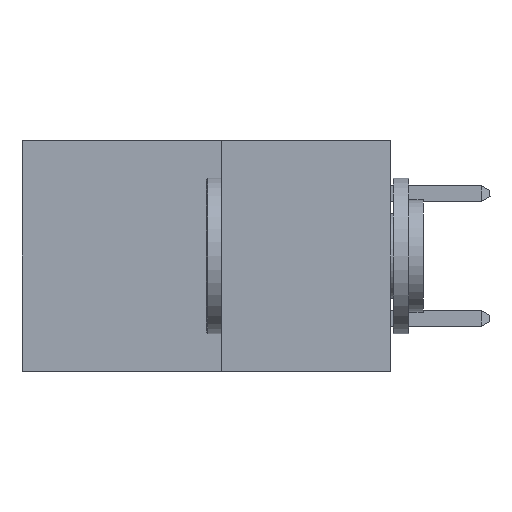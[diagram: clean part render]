
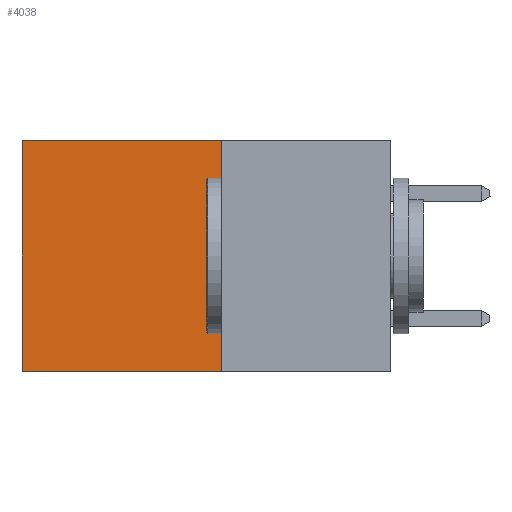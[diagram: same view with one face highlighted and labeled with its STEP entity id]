
A CAD part, left-side view. The second image highlights one B-rep face of the part: STEP entity #4038.
In plain terms, the highlighted planar face has unit normal (-1, 0, 0).
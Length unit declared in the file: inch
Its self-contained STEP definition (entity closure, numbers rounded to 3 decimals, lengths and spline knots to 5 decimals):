
#106 = CARTESIAN_POINT ( 'NONE',  ( 0.277, 0.27, 0. ) ) ;
#131 = FACE_OUTER_BOUND ( 'NONE', #7507, .T. ) ;
#417 = VECTOR ( 'NONE', #4215, 39.37008 ) ;
#595 = CARTESIAN_POINT ( 'NONE',  ( 0.277, 0.27, -0.37 ) ) ;
#642 = LINE ( 'NONE', #595, #4443 ) ;
#970 = DIRECTION ( 'NONE',  ( 0., 0., -1. ) ) ;
#993 = DIRECTION ( 'NONE',  ( 0., 1., 0. ) ) ;
#1677 = VERTEX_POINT ( 'NONE', #7976 ) ;
#2417 = DIRECTION ( 'NONE',  ( 0., 0., -1. ) ) ;
#2466 = DIRECTION ( 'NONE',  ( 1., 0., 0. ) ) ;
#2573 = PLANE ( 'NONE',  #6411 ) ;
#2604 = CARTESIAN_POINT ( 'NONE',  ( 0.277, 0.27, -0.37 ) ) ;
#2623 = EDGE_CURVE ( 'NONE', #2734, #1677, #4226, .T. ) ;
#2656 = ORIENTED_EDGE ( 'NONE', *, *, #5081, .F. ) ;
#2734 = VERTEX_POINT ( 'NONE', #5422 ) ;
#2770 = LINE ( 'NONE', #3308, #3001 ) ;
#2946 = ORIENTED_EDGE ( 'NONE', *, *, #2623, .T. ) ;
#3001 = VECTOR ( 'NONE', #3415, 39.37008 ) ;
#3308 = CARTESIAN_POINT ( 'NONE',  ( 0.277, 0.27, 0. ) ) ;
#3415 = DIRECTION ( 'NONE',  ( 0., 1., 0. ) ) ;
#3987 = VECTOR ( 'NONE', #993, 39.37008 ) ;
#4038 = ADVANCED_FACE ( 'NONE', ( #131 ), #2573, .F. ) ;
#4169 = CARTESIAN_POINT ( 'NONE',  ( 0.277, 0.59, -0.37 ) ) ;
#4215 = DIRECTION ( 'NONE',  ( 0., 0., -1. ) ) ;
#4226 = LINE ( 'NONE', #4169, #417 ) ;
#4443 = VECTOR ( 'NONE', #970, 39.37008 ) ;
#4773 = ORIENTED_EDGE ( 'NONE', *, *, #6173, .F. ) ;
#5081 = EDGE_CURVE ( 'NONE', #5154, #1677, #6202, .T. ) ;
#5154 = VERTEX_POINT ( 'NONE', #7592 ) ;
#5422 = CARTESIAN_POINT ( 'NONE',  ( 0.277, 0.59, 0. ) ) ;
#5450 = EDGE_CURVE ( 'NONE', #6289, #2734, #2770, .T. ) ;
#6173 = EDGE_CURVE ( 'NONE', #6289, #5154, #642, .T. ) ;
#6202 = LINE ( 'NONE', #8114, #3987 ) ;
#6289 = VERTEX_POINT ( 'NONE', #106 ) ;
#6411 = AXIS2_PLACEMENT_3D ( 'NONE', #2604, #2466, #2417 ) ;
#7507 = EDGE_LOOP ( 'NONE', ( #2946, #2656, #4773, #8731 ) ) ;
#7592 = CARTESIAN_POINT ( 'NONE',  ( 0.277, 0.27, -0.37 ) ) ;
#7976 = CARTESIAN_POINT ( 'NONE',  ( 0.277, 0.59, -0.37 ) ) ;
#8114 = CARTESIAN_POINT ( 'NONE',  ( 0.277, 0.27, -0.37 ) ) ;
#8731 = ORIENTED_EDGE ( 'NONE', *, *, #5450, .T. ) ;
